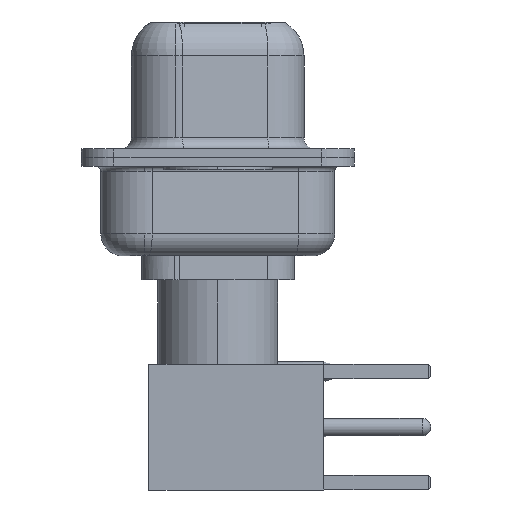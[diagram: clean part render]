
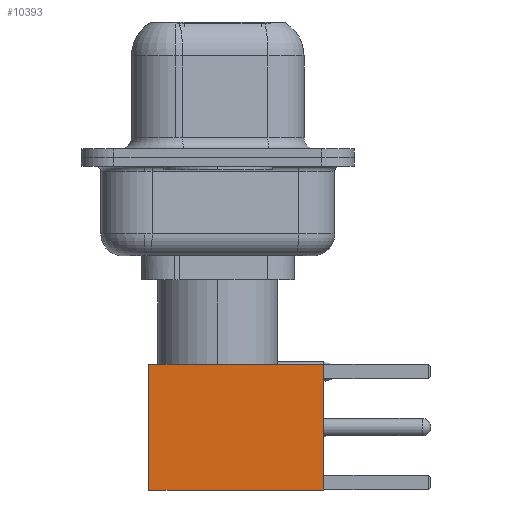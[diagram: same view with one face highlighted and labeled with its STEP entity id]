
A CAD part, left-side view. The second image highlights one B-rep face of the part: STEP entity #10393.
In plain terms, the highlighted face is planar.
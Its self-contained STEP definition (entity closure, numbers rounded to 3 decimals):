
#122 = VECTOR ( 'NONE', #13396, 1000. ) ;
#263 = DIRECTION ( 'NONE',  ( -1., 0., 0. ) ) ;
#462 = LINE ( 'NONE', #14306, #122 ) ;
#789 = EDGE_CURVE ( 'NONE', #17241, #16256, #12398, .T. ) ;
#1257 = EDGE_CURVE ( 'NONE', #3982, #16256, #462, .T. ) ;
#3662 = VECTOR ( 'NONE', #13879, 1000. ) ;
#3775 = CARTESIAN_POINT ( 'NONE',  ( -2.875, 2.875, 0. ) ) ;
#3982 = VERTEX_POINT ( 'NONE', #21746 ) ;
#4965 = CARTESIAN_POINT ( 'NONE',  ( 2.875, 2.875, 0. ) ) ;
#5149 = ORIENTED_EDGE ( 'NONE', *, *, #19644, .T. ) ;
#6461 = DIRECTION ( 'NONE',  ( 0., 0., 1. ) ) ;
#7112 = CARTESIAN_POINT ( 'NONE',  ( -2.875, 2.875, 8. ) ) ;
#7303 = LINE ( 'NONE', #8997, #8885 ) ;
#7790 = ORIENTED_EDGE ( 'NONE', *, *, #789, .F. ) ;
#7836 = AXIS2_PLACEMENT_3D ( 'NONE', #4965, #9748, #6461 ) ;
#8485 = PLANE ( 'NONE',  #7836 ) ;
#8885 = VECTOR ( 'NONE', #263, 1000. ) ;
#8997 = CARTESIAN_POINT ( 'NONE',  ( 0., 2.875, 8. ) ) ;
#9283 = EDGE_CURVE ( 'NONE', #19977, #17241, #7303, .T. ) ;
#9545 = ORIENTED_EDGE ( 'NONE', *, *, #9283, .F. ) ;
#9748 = DIRECTION ( 'NONE',  ( 0., 1., 0. ) ) ;
#10231 = CARTESIAN_POINT ( 'NONE',  ( 2.875, 2.875, 0. ) ) ;
#10393 = ADVANCED_FACE ( 'NONE', ( #18845 ), #8485, .T. ) ;
#10684 = DIRECTION ( 'NONE',  ( 0., 0., -1. ) ) ;
#11057 = VECTOR ( 'NONE', #10684, 1000. ) ;
#11128 = CARTESIAN_POINT ( 'NONE',  ( 2.875, 2.875, 8. ) ) ;
#12398 = LINE ( 'NONE', #3775, #11057 ) ;
#12745 = EDGE_LOOP ( 'NONE', ( #5149, #20672, #7790, #9545 ) ) ;
#13396 = DIRECTION ( 'NONE',  ( -1., 0., 0. ) ) ;
#13879 = DIRECTION ( 'NONE',  ( 0., 0., -1. ) ) ;
#14306 = CARTESIAN_POINT ( 'NONE',  ( 0., 2.875, 0. ) ) ;
#16256 = VERTEX_POINT ( 'NONE', #17411 ) ;
#17241 = VERTEX_POINT ( 'NONE', #7112 ) ;
#17411 = CARTESIAN_POINT ( 'NONE',  ( -2.875, 2.875, 0. ) ) ;
#17415 = LINE ( 'NONE', #10231, #3662 ) ;
#18845 = FACE_OUTER_BOUND ( 'NONE', #12745, .T. ) ;
#19644 = EDGE_CURVE ( 'NONE', #19977, #3982, #17415, .T. ) ;
#19977 = VERTEX_POINT ( 'NONE', #11128 ) ;
#20672 = ORIENTED_EDGE ( 'NONE', *, *, #1257, .T. ) ;
#21746 = CARTESIAN_POINT ( 'NONE',  ( 2.875, 2.875, 0. ) ) ;
